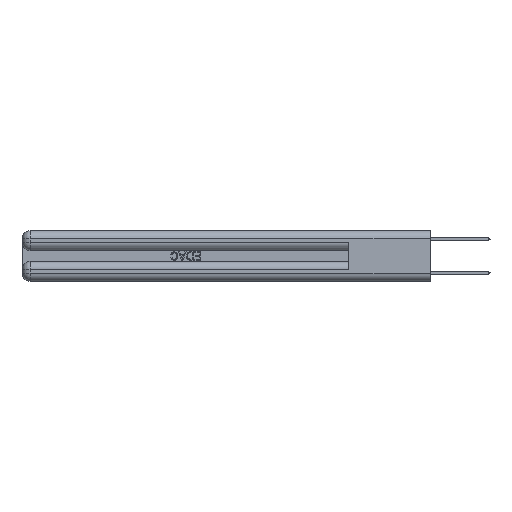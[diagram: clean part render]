
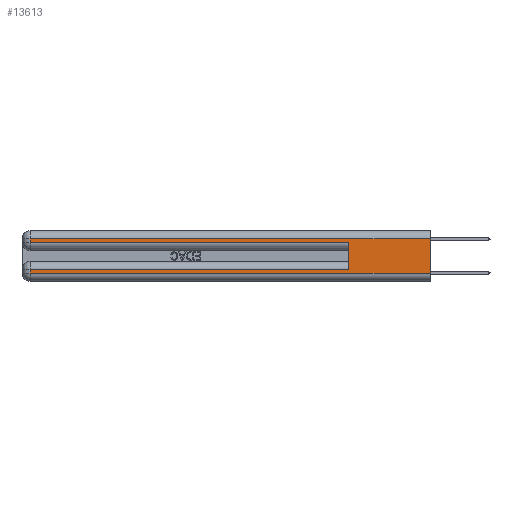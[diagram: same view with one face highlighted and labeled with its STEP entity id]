
A CAD part, left-side view. The second image highlights one B-rep face of the part: STEP entity #13613.
In plain terms, the highlighted planar face has unit normal (-1, 0, 0).
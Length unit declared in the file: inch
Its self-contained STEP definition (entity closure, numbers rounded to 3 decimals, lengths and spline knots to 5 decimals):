
#52 = DIRECTION ( 'NONE',  ( 0., -1., 0. ) ) ;
#588 = VECTOR ( 'NONE', #32799, 39.37008 ) ;
#1050 = CARTESIAN_POINT ( 'NONE',  ( 0., 0., 0.085 ) ) ;
#1531 = CARTESIAN_POINT ( 'NONE',  ( 0., 0., 0.31 ) ) ;
#1558 = EDGE_CURVE ( 'NONE', #22982, #7171, #24248, .T. ) ;
#3017 = VERTEX_POINT ( 'NONE', #26748 ) ;
#5389 = CARTESIAN_POINT ( 'NONE',  ( 0., 2.94, 0.37 ) ) ;
#5410 = CARTESIAN_POINT ( 'NONE',  ( 0., 0.6, 0.145 ) ) ;
#6333 = ORIENTED_EDGE ( 'NONE', *, *, #6483, .T. ) ;
#6483 = EDGE_CURVE ( 'NONE', #7715, #7171, #24166, .T. ) ;
#6632 = ORIENTED_EDGE ( 'NONE', *, *, #33495, .T. ) ;
#7171 = VERTEX_POINT ( 'NONE', #21073 ) ;
#7200 = VERTEX_POINT ( 'NONE', #34296 ) ;
#7293 = EDGE_CURVE ( 'NONE', #10829, #18419, #18230, .T. ) ;
#7715 = VERTEX_POINT ( 'NONE', #23829 ) ;
#7887 = DIRECTION ( 'NONE',  ( 0., 0., -1. ) ) ;
#8755 = PLANE ( 'NONE',  #27600 ) ;
#8926 = FACE_OUTER_BOUND ( 'NONE', #15847, .T. ) ;
#10016 = VECTOR ( 'NONE', #29101, 39.37008 ) ;
#10207 = VERTEX_POINT ( 'NONE', #18446 ) ;
#10829 = VERTEX_POINT ( 'NONE', #27289 ) ;
#11272 = EDGE_CURVE ( 'NONE', #22982, #10207, #25392, .T. ) ;
#12046 = LINE ( 'NONE', #27234, #26129 ) ;
#12192 = ORIENTED_EDGE ( 'NONE', *, *, #12504, .F. ) ;
#12504 = EDGE_CURVE ( 'NONE', #10829, #3017, #16754, .T. ) ;
#13613 = ADVANCED_FACE ( 'NONE', ( #8926 ), #8755, .F. ) ;
#13885 = ORIENTED_EDGE ( 'NONE', *, *, #7293, .T. ) ;
#14354 = VECTOR ( 'NONE', #7887, 39.37008 ) ;
#14615 = VECTOR ( 'NONE', #33148, 39.37008 ) ;
#15521 = ORIENTED_EDGE ( 'NONE', *, *, #1558, .F. ) ;
#15847 = EDGE_LOOP ( 'NONE', ( #12192, #13885, #20488, #6333, #15521, #32885, #16575, #6632 ) ) ;
#16170 = CARTESIAN_POINT ( 'NONE',  ( 0., 0., 0.285 ) ) ;
#16575 = ORIENTED_EDGE ( 'NONE', *, *, #29155, .T. ) ;
#16754 = LINE ( 'NONE', #30616, #14615 ) ;
#17391 = DIRECTION ( 'NONE',  ( 0., 1., 0. ) ) ;
#18230 = LINE ( 'NONE', #1531, #10016 ) ;
#18419 = VERTEX_POINT ( 'NONE', #33525 ) ;
#18446 = CARTESIAN_POINT ( 'NONE',  ( 0., 2.94, 0.085 ) ) ;
#20488 = ORIENTED_EDGE ( 'NONE', *, *, #25205, .T. ) ;
#21073 = CARTESIAN_POINT ( 'NONE',  ( 0., 0.6, 0.285 ) ) ;
#21645 = CARTESIAN_POINT ( 'NONE',  ( 0., 0.6, 0.085 ) ) ;
#22607 = DIRECTION ( 'NONE',  ( 0., 0., -1. ) ) ;
#22982 = VERTEX_POINT ( 'NONE', #21645 ) ;
#23829 = CARTESIAN_POINT ( 'NONE',  ( 0., 2.94, 0.285 ) ) ;
#24166 = LINE ( 'NONE', #16170, #29933 ) ;
#24248 = LINE ( 'NONE', #5410, #588 ) ;
#24573 = DIRECTION ( 'NONE',  ( 1., 0., 0. ) ) ;
#25048 = DIRECTION ( 'NONE',  ( 0., -1., 0. ) ) ;
#25092 = CARTESIAN_POINT ( 'NONE',  ( 0., 0., 0.37 ) ) ;
#25205 = EDGE_CURVE ( 'NONE', #18419, #7715, #29590, .T. ) ;
#25392 = LINE ( 'NONE', #1050, #29168 ) ;
#26129 = VECTOR ( 'NONE', #52, 39.37008 ) ;
#26748 = CARTESIAN_POINT ( 'NONE',  ( 0., 0., 0.06 ) ) ;
#27234 = CARTESIAN_POINT ( 'NONE',  ( 0., 0., 0.06 ) ) ;
#27289 = CARTESIAN_POINT ( 'NONE',  ( 0., 0., 0.31 ) ) ;
#27600 = AXIS2_PLACEMENT_3D ( 'NONE', #25092, #24573, #22607 ) ;
#29101 = DIRECTION ( 'NONE',  ( 0., 1., 0. ) ) ;
#29155 = EDGE_CURVE ( 'NONE', #10207, #7200, #33169, .T. ) ;
#29168 = VECTOR ( 'NONE', #17391, 39.37008 ) ;
#29590 = LINE ( 'NONE', #5389, #14354 ) ;
#29933 = VECTOR ( 'NONE', #25048, 39.37008 ) ;
#30616 = CARTESIAN_POINT ( 'NONE',  ( 0., 0., 0.37 ) ) ;
#32635 = CARTESIAN_POINT ( 'NONE',  ( 0., 2.94, 0.37 ) ) ;
#32799 = DIRECTION ( 'NONE',  ( 0., 0., 1. ) ) ;
#32805 = DIRECTION ( 'NONE',  ( 0., 0., -1. ) ) ;
#32885 = ORIENTED_EDGE ( 'NONE', *, *, #11272, .T. ) ;
#33148 = DIRECTION ( 'NONE',  ( 0., 0., -1. ) ) ;
#33169 = LINE ( 'NONE', #32635, #34379 ) ;
#33495 = EDGE_CURVE ( 'NONE', #7200, #3017, #12046, .T. ) ;
#33525 = CARTESIAN_POINT ( 'NONE',  ( 0., 2.94, 0.31 ) ) ;
#34296 = CARTESIAN_POINT ( 'NONE',  ( 0., 2.94, 0.06 ) ) ;
#34379 = VECTOR ( 'NONE', #32805, 39.37008 ) ;
